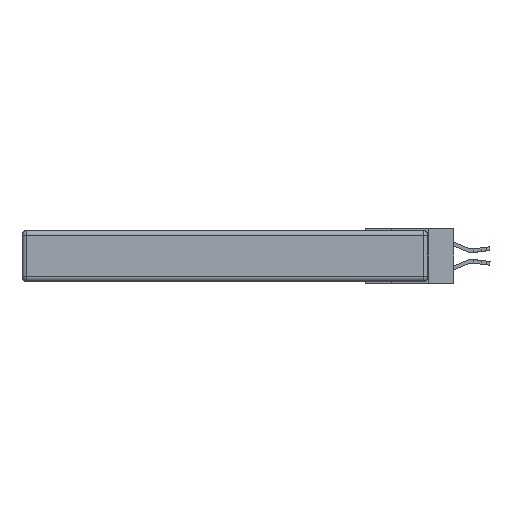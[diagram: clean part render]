
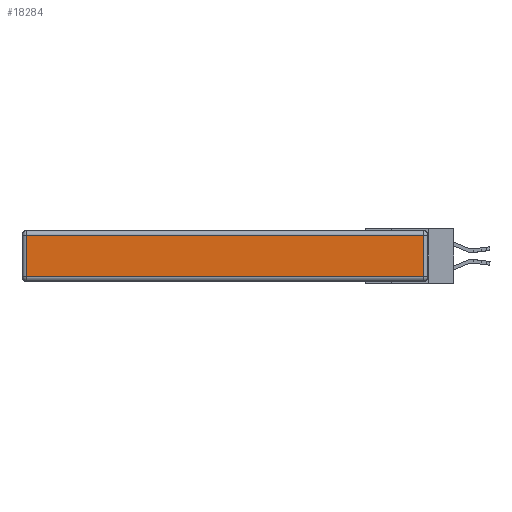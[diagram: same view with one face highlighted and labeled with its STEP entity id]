
A CAD part, left-side view. The second image highlights one B-rep face of the part: STEP entity #18284.
In plain terms, the highlighted planar face has unit normal (-1, 0, 0).
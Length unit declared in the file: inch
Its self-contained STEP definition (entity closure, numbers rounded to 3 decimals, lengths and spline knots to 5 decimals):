
#351 = VECTOR ( 'NONE', #16514, 39.37008 ) ;
#1499 = CARTESIAN_POINT ( 'NONE',  ( 0., 0., -0.343 ) ) ;
#2208 = CARTESIAN_POINT ( 'NONE',  ( 0., 0., -0.313 ) ) ;
#2446 = EDGE_CURVE ( 'NONE', #17415, #2668, #6197, .T. ) ;
#2668 = VERTEX_POINT ( 'NONE', #9261 ) ;
#3709 = CARTESIAN_POINT ( 'NONE',  ( 0., 2.75, -0.03 ) ) ;
#3985 = EDGE_LOOP ( 'NONE', ( #10155, #9078, #18289, #6865 ) ) ;
#4633 = DIRECTION ( 'NONE',  ( 0., 0., 1. ) ) ;
#4845 = CARTESIAN_POINT ( 'NONE',  ( 0., 2.72, -0.343 ) ) ;
#5777 = LINE ( 'NONE', #17989, #351 ) ;
#5961 = DIRECTION ( 'NONE',  ( 0., 0., -1. ) ) ;
#6197 = LINE ( 'NONE', #2208, #16992 ) ;
#6865 = ORIENTED_EDGE ( 'NONE', *, *, #7313, .T. ) ;
#6880 = DIRECTION ( 'NONE',  ( 0., 1., 0. ) ) ;
#7313 = EDGE_CURVE ( 'NONE', #15618, #17415, #19092, .T. ) ;
#9078 = ORIENTED_EDGE ( 'NONE', *, *, #13089, .T. ) ;
#9261 = CARTESIAN_POINT ( 'NONE',  ( 0., 0.03, -0.313 ) ) ;
#10069 = LINE ( 'NONE', #3709, #20069 ) ;
#10155 = ORIENTED_EDGE ( 'NONE', *, *, #2446, .T. ) ;
#11724 = AXIS2_PLACEMENT_3D ( 'NONE', #1499, #14051, #4633 ) ;
#11733 = DIRECTION ( 'NONE',  ( 0., -1., 0. ) ) ;
#12402 = PLANE ( 'NONE',  #11724 ) ;
#13089 = EDGE_CURVE ( 'NONE', #2668, #16228, #5777, .T. ) ;
#14051 = DIRECTION ( 'NONE',  ( -1., 0., 0. ) ) ;
#15618 = VERTEX_POINT ( 'NONE', #18595 ) ;
#16228 = VERTEX_POINT ( 'NONE', #17350 ) ;
#16514 = DIRECTION ( 'NONE',  ( 0., 0., 1. ) ) ;
#16992 = VECTOR ( 'NONE', #11733, 39.37008 ) ;
#17124 = EDGE_CURVE ( 'NONE', #16228, #15618, #10069, .T. ) ;
#17139 = CARTESIAN_POINT ( 'NONE',  ( 0., 2.72, -0.313 ) ) ;
#17350 = CARTESIAN_POINT ( 'NONE',  ( 0., 0.03, -0.03 ) ) ;
#17415 = VERTEX_POINT ( 'NONE', #17139 ) ;
#17631 = VECTOR ( 'NONE', #5961, 39.37008 ) ;
#17989 = CARTESIAN_POINT ( 'NONE',  ( 0., 0.03, -0.343 ) ) ;
#18284 = ADVANCED_FACE ( 'NONE', ( #18787 ), #12402, .T. ) ;
#18289 = ORIENTED_EDGE ( 'NONE', *, *, #17124, .T. ) ;
#18595 = CARTESIAN_POINT ( 'NONE',  ( 0., 2.72, -0.03 ) ) ;
#18787 = FACE_OUTER_BOUND ( 'NONE', #3985, .T. ) ;
#19092 = LINE ( 'NONE', #4845, #17631 ) ;
#20069 = VECTOR ( 'NONE', #6880, 39.37008 ) ;
